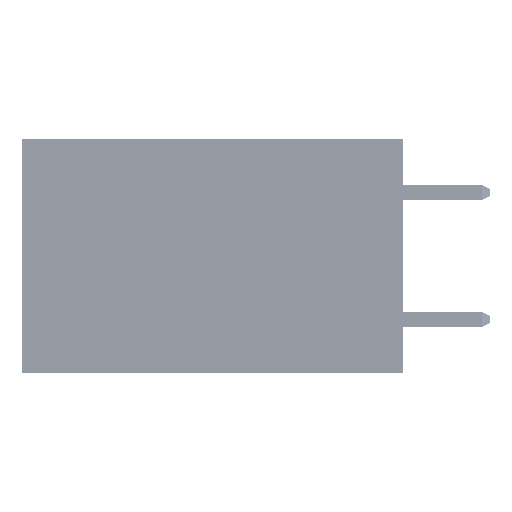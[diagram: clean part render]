
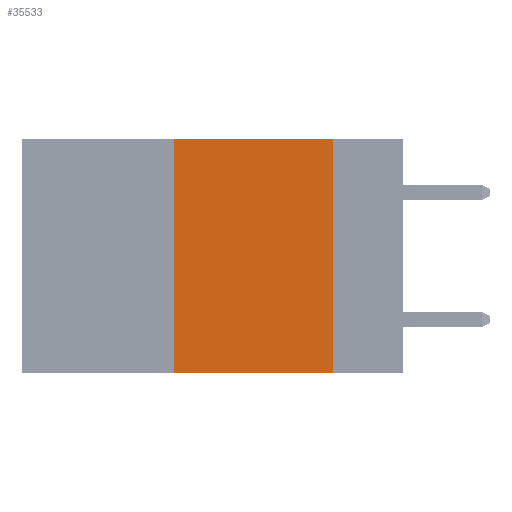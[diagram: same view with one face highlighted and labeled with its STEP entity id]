
A CAD part, left-side view. The second image highlights one B-rep face of the part: STEP entity #35533.
In plain terms, the highlighted planar face has unit normal (-1, 0, 0).
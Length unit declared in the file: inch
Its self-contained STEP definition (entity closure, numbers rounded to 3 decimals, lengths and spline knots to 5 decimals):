
#2469 = EDGE_CURVE ( 'NONE', #29596, #18067, #3110, .T. ) ;
#2655 = DIRECTION ( 'NONE',  ( 1., 0., 0. ) ) ;
#2772 = CARTESIAN_POINT ( 'NONE',  ( 0., 0.36, 0. ) ) ;
#3030 = LINE ( 'NONE', #2772, #8630 ) ;
#3085 = LINE ( 'NONE', #36518, #27162 ) ;
#3110 = LINE ( 'NONE', #6690, #20639 ) ;
#4821 = CARTESIAN_POINT ( 'NONE',  ( 0., 0.11, -0.37 ) ) ;
#5128 = DIRECTION ( 'NONE',  ( 0., 0., -1. ) ) ;
#5228 = CARTESIAN_POINT ( 'NONE',  ( 0., 0.36, 0. ) ) ;
#6690 = CARTESIAN_POINT ( 'NONE',  ( 0., 0.11, 0. ) ) ;
#8630 = VECTOR ( 'NONE', #10680, 39.37008 ) ;
#8897 = CARTESIAN_POINT ( 'NONE',  ( 0., 0.6, 0. ) ) ;
#10680 = DIRECTION ( 'NONE',  ( 0., 0., 1. ) ) ;
#12641 = AXIS2_PLACEMENT_3D ( 'NONE', #17011, #2655, #5128 ) ;
#14085 = DIRECTION ( 'NONE',  ( 0., -1., 0. ) ) ;
#14896 = CARTESIAN_POINT ( 'NONE',  ( 0., 0.36, -0.37 ) ) ;
#15321 = VERTEX_POINT ( 'NONE', #5228 ) ;
#17011 = CARTESIAN_POINT ( 'NONE',  ( 0., 0.6, 0. ) ) ;
#18067 = VERTEX_POINT ( 'NONE', #4821 ) ;
#19083 = ORIENTED_EDGE ( 'NONE', *, *, #34112, .F. ) ;
#19492 = FACE_OUTER_BOUND ( 'NONE', #21432, .T. ) ;
#20639 = VECTOR ( 'NONE', #36296, 39.37008 ) ;
#21432 = EDGE_LOOP ( 'NONE', ( #25432, #19083, #39027, #28468 ) ) ;
#23019 = DIRECTION ( 'NONE',  ( 0., -1., 0. ) ) ;
#23315 = EDGE_CURVE ( 'NONE', #41268, #15321, #3030, .T. ) ;
#25432 = ORIENTED_EDGE ( 'NONE', *, *, #2469, .F. ) ;
#26717 = EDGE_CURVE ( 'NONE', #41268, #18067, #3085, .T. ) ;
#27162 = VECTOR ( 'NONE', #14085, 39.37008 ) ;
#27977 = PLANE ( 'NONE',  #12641 ) ;
#28468 = ORIENTED_EDGE ( 'NONE', *, *, #26717, .T. ) ;
#29596 = VERTEX_POINT ( 'NONE', #42499 ) ;
#34112 = EDGE_CURVE ( 'NONE', #15321, #29596, #41638, .T. ) ;
#35533 = ADVANCED_FACE ( 'NONE', ( #19492 ), #27977, .F. ) ;
#36296 = DIRECTION ( 'NONE',  ( 0., 0., -1. ) ) ;
#36518 = CARTESIAN_POINT ( 'NONE',  ( 0., 0.6, -0.37 ) ) ;
#39027 = ORIENTED_EDGE ( 'NONE', *, *, #23315, .F. ) ;
#41268 = VERTEX_POINT ( 'NONE', #14896 ) ;
#41638 = LINE ( 'NONE', #8897, #46125 ) ;
#42499 = CARTESIAN_POINT ( 'NONE',  ( 0., 0.11, 0. ) ) ;
#46125 = VECTOR ( 'NONE', #23019, 39.37008 ) ;
